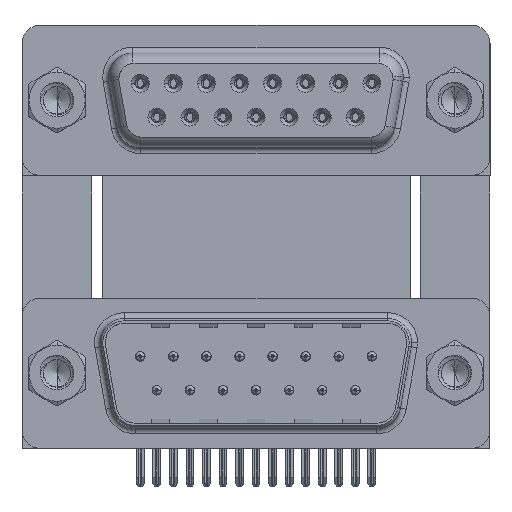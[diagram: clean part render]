
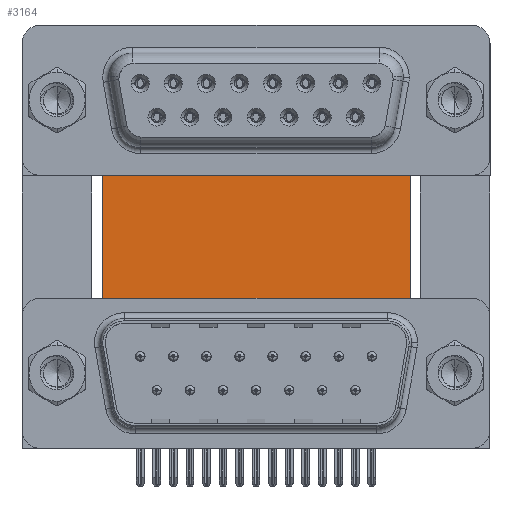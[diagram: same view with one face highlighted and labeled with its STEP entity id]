
A CAD part, top view. The second image highlights one B-rep face of the part: STEP entity #3164.
In plain terms, the highlighted planar face has unit normal (0, 0, 1).
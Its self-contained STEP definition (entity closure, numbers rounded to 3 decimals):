
#317 = LINE ( 'NONE', #4016, #936 ) ;
#804 = CARTESIAN_POINT ( 'NONE',  ( 29.58, 16.585, -12. ) ) ;
#936 = VECTOR ( 'NONE', #19821, 1000. ) ;
#3164 = ADVANCED_FACE ( 'NONE', ( #3288 ), #18367, .F. ) ;
#3205 = ORIENTED_EDGE ( 'NONE', *, *, #13702, .F. ) ;
#3288 = FACE_OUTER_BOUND ( 'NONE', #16969, .T. ) ;
#4015 = CARTESIAN_POINT ( 'NONE',  ( 3.79, 16.585, -12. ) ) ;
#4016 = CARTESIAN_POINT ( 'NONE',  ( 3.79, 16.585, -12. ) ) ;
#4606 = CARTESIAN_POINT ( 'NONE',  ( 3.79, -3.735, -12. ) ) ;
#12579 = CARTESIAN_POINT ( 'NONE',  ( 29.58, 16.585, -12. ) ) ;
#12607 = DIRECTION ( 'NONE',  ( 1., 0., 0. ) ) ;
#13702 = EDGE_CURVE ( 'NONE', #28348, #24756, #27425, .T. ) ;
#13805 = CARTESIAN_POINT ( 'NONE',  ( 29.58, -3.735, -12. ) ) ;
#14680 = ORIENTED_EDGE ( 'NONE', *, *, #25107, .T. ) ;
#16636 = CARTESIAN_POINT ( 'NONE',  ( 3.79, 16.585, -12. ) ) ;
#16969 = EDGE_LOOP ( 'NONE', ( #14680, #46899, #3205, #36956 ) ) ;
#18367 = PLANE ( 'NONE',  #40943 ) ;
#18969 = LINE ( 'NONE', #4606, #44222 ) ;
#19299 = CARTESIAN_POINT ( 'NONE',  ( 3.79, 16.585, -12. ) ) ;
#19821 = DIRECTION ( 'NONE',  ( 0., -1., 0. ) ) ;
#20300 = VECTOR ( 'NONE', #34416, 1000. ) ;
#23174 = VECTOR ( 'NONE', #12607, 1000. ) ;
#24756 = VERTEX_POINT ( 'NONE', #12579 ) ;
#25107 = EDGE_CURVE ( 'NONE', #35734, #41229, #18969, .T. ) ;
#26730 = CARTESIAN_POINT ( 'NONE',  ( 3.79, -3.735, -12. ) ) ;
#26854 = DIRECTION ( 'NONE',  ( 1., 0., 0. ) ) ;
#27425 = LINE ( 'NONE', #19299, #23174 ) ;
#28348 = VERTEX_POINT ( 'NONE', #16636 ) ;
#34416 = DIRECTION ( 'NONE',  ( 0., -1., 0. ) ) ;
#35734 = VERTEX_POINT ( 'NONE', #26730 ) ;
#36956 = ORIENTED_EDGE ( 'NONE', *, *, #37850, .T. ) ;
#37850 = EDGE_CURVE ( 'NONE', #28348, #35734, #317, .T. ) ;
#39889 = EDGE_CURVE ( 'NONE', #24756, #41229, #46256, .T. ) ;
#40943 = AXIS2_PLACEMENT_3D ( 'NONE', #4015, #48495, #47998 ) ;
#41229 = VERTEX_POINT ( 'NONE', #13805 ) ;
#44222 = VECTOR ( 'NONE', #26854, 1000. ) ;
#46256 = LINE ( 'NONE', #804, #20300 ) ;
#46899 = ORIENTED_EDGE ( 'NONE', *, *, #39889, .F. ) ;
#47998 = DIRECTION ( 'NONE',  ( -1., 0., 0. ) ) ;
#48495 = DIRECTION ( 'NONE',  ( 0., 0., -1. ) ) ;
